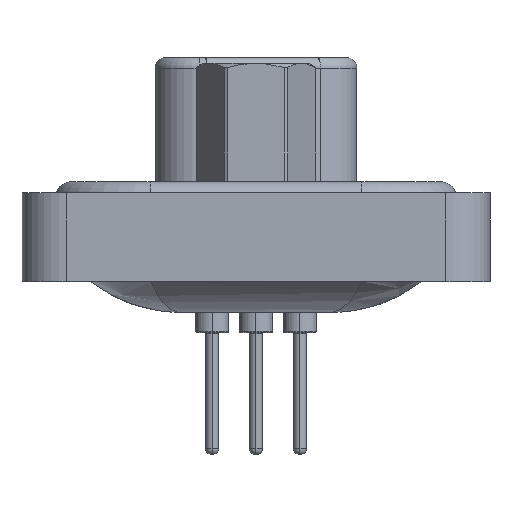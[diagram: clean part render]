
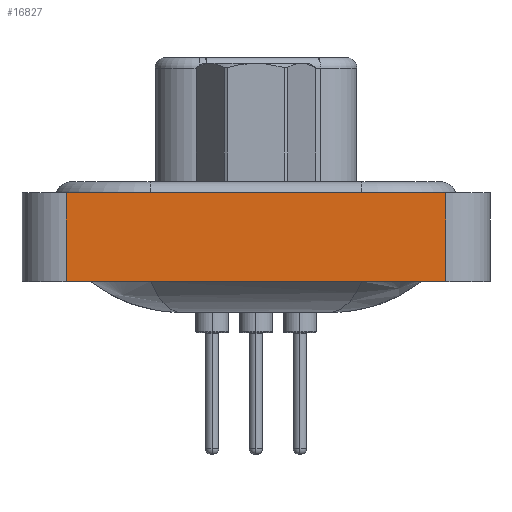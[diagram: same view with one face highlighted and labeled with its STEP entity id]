
A CAD part, left-side view. The second image highlights one B-rep face of the part: STEP entity #16827.
In plain terms, the highlighted planar face has unit normal (-1, 0, 0).
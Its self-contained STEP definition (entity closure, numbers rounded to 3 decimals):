
#2553 = FACE_OUTER_BOUND ( 'NONE', #9747, .T. ) ;
#3195 = PLANE ( 'NONE',  #20062 ) ;
#3233 = VERTEX_POINT ( 'NONE', #10133 ) ;
#3656 = CARTESIAN_POINT ( 'NONE',  ( -7.35, -8.55, -3.6 ) ) ;
#5928 = DIRECTION ( 'NONE',  ( -1., 0., 0. ) ) ;
#6398 = DIRECTION ( 'NONE',  ( 0., 0., 1. ) ) ;
#7313 = CARTESIAN_POINT ( 'NONE',  ( -7.35, -8.55, 0.4 ) ) ;
#7993 = VERTEX_POINT ( 'NONE', #7313 ) ;
#9547 = VECTOR ( 'NONE', #18696, 1000. ) ;
#9747 = EDGE_LOOP ( 'NONE', ( #26177, #22534, #19185, #16700 ) ) ;
#10133 = CARTESIAN_POINT ( 'NONE',  ( -7.35, 8.55, 0.4 ) ) ;
#10342 = CARTESIAN_POINT ( 'NONE',  ( -7.35, 8.55, -3.6 ) ) ;
#10420 = LINE ( 'NONE', #21467, #9547 ) ;
#10842 = LINE ( 'NONE', #3656, #20836 ) ;
#10948 = DIRECTION ( 'NONE',  ( 0., -1., 0. ) ) ;
#11155 = LINE ( 'NONE', #29953, #25616 ) ;
#11695 = CARTESIAN_POINT ( 'NONE',  ( -7.35, 8.55, -3.6 ) ) ;
#13903 = VERTEX_POINT ( 'NONE', #10342 ) ;
#14427 = DIRECTION ( 'NONE',  ( 0., 0., 1. ) ) ;
#16700 = ORIENTED_EDGE ( 'NONE', *, *, #31521, .T. ) ;
#16827 = ADVANCED_FACE ( 'NONE', ( #2553 ), #3195, .T. ) ;
#16955 = EDGE_CURVE ( 'NONE', #25940, #7993, #10842, .T. ) ;
#18696 = DIRECTION ( 'NONE',  ( 0., -1., 0. ) ) ;
#19185 = ORIENTED_EDGE ( 'NONE', *, *, #29697, .F. ) ;
#19489 = CARTESIAN_POINT ( 'NONE',  ( -7.35, -8.55, -3.6 ) ) ;
#20062 = AXIS2_PLACEMENT_3D ( 'NONE', #19489, #5928, #24975 ) ;
#20836 = VECTOR ( 'NONE', #6398, 1000. ) ;
#21467 = CARTESIAN_POINT ( 'NONE',  ( -7.35, -8.55, -3.6 ) ) ;
#22534 = ORIENTED_EDGE ( 'NONE', *, *, #24275, .F. ) ;
#24275 = EDGE_CURVE ( 'NONE', #3233, #7993, #11155, .T. ) ;
#24975 = DIRECTION ( 'NONE',  ( 0., 0., 1. ) ) ;
#25616 = VECTOR ( 'NONE', #10948, 1000. ) ;
#25940 = VERTEX_POINT ( 'NONE', #27096 ) ;
#26177 = ORIENTED_EDGE ( 'NONE', *, *, #16955, .T. ) ;
#27096 = CARTESIAN_POINT ( 'NONE',  ( -7.35, -8.55, -3.6 ) ) ;
#27528 = LINE ( 'NONE', #11695, #32222 ) ;
#29697 = EDGE_CURVE ( 'NONE', #13903, #3233, #27528, .T. ) ;
#29953 = CARTESIAN_POINT ( 'NONE',  ( -7.35, -8.55, 0.4 ) ) ;
#31521 = EDGE_CURVE ( 'NONE', #13903, #25940, #10420, .T. ) ;
#32222 = VECTOR ( 'NONE', #14427, 1000. ) ;
